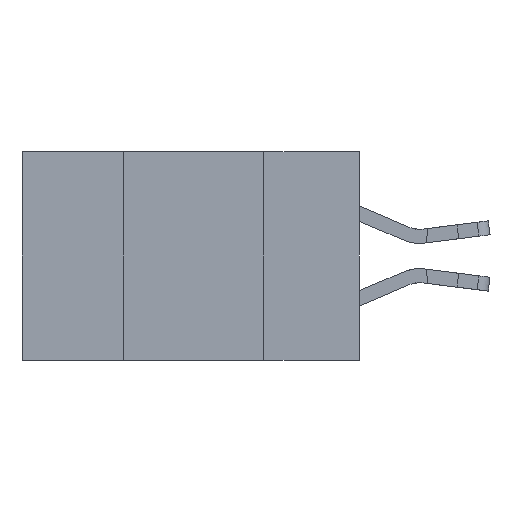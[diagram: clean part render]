
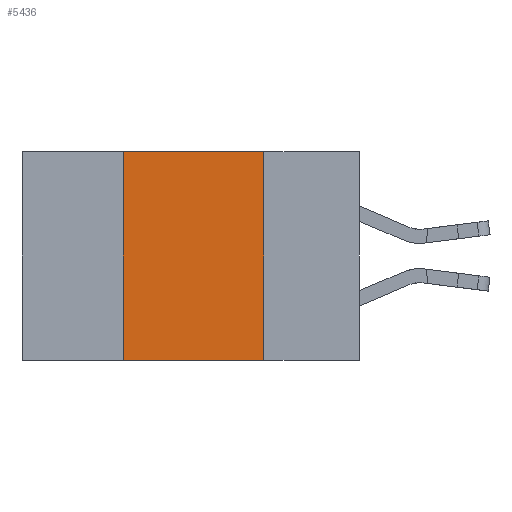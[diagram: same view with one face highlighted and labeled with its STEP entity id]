
A CAD part, left-side view. The second image highlights one B-rep face of the part: STEP entity #5436.
In plain terms, the highlighted planar face has unit normal (-1, 0, 0).
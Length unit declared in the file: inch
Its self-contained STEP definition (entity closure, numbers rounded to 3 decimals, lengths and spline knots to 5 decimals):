
#478 = CARTESIAN_POINT ( 'NONE',  ( 0., 0.17, -0.37 ) ) ;
#2420 = AXIS2_PLACEMENT_3D ( 'NONE', #10141, #10089, #15312 ) ;
#3074 = LINE ( 'NONE', #9071, #9560 ) ;
#3492 = CARTESIAN_POINT ( 'NONE',  ( 0., 0.42, -0.37 ) ) ;
#3863 = VECTOR ( 'NONE', #12169, 39.37008 ) ;
#4345 = EDGE_CURVE ( 'NONE', #14969, #10926, #3074, .T. ) ;
#5436 = ADVANCED_FACE ( 'NONE', ( #9960 ), #6864, .F. ) ;
#5813 = DIRECTION ( 'NONE',  ( 0., 0., -1. ) ) ;
#5998 = DIRECTION ( 'NONE',  ( 0., 0., 1. ) ) ;
#6363 = EDGE_CURVE ( 'NONE', #10428, #10926, #6857, .T. ) ;
#6839 = LINE ( 'NONE', #10558, #16037 ) ;
#6857 = LINE ( 'NONE', #7007, #3863 ) ;
#6864 = PLANE ( 'NONE',  #2420 ) ;
#6871 = EDGE_CURVE ( 'NONE', #11516, #14969, #6839, .T. ) ;
#7007 = CARTESIAN_POINT ( 'NONE',  ( 0., 0.6, -0.37 ) ) ;
#7735 = VECTOR ( 'NONE', #5998, 39.37008 ) ;
#8259 = CARTESIAN_POINT ( 'NONE',  ( 0., 0.17, 0. ) ) ;
#8646 = EDGE_LOOP ( 'NONE', ( #16294, #10387, #9596, #15036 ) ) ;
#9071 = CARTESIAN_POINT ( 'NONE',  ( 0., 0.17, 0. ) ) ;
#9256 = DIRECTION ( 'NONE',  ( 0., -1., 0. ) ) ;
#9560 = VECTOR ( 'NONE', #5813, 39.37008 ) ;
#9596 = ORIENTED_EDGE ( 'NONE', *, *, #9748, .F. ) ;
#9748 = EDGE_CURVE ( 'NONE', #10428, #11516, #11154, .T. ) ;
#9960 = FACE_OUTER_BOUND ( 'NONE', #8646, .T. ) ;
#10089 = DIRECTION ( 'NONE',  ( 1., 0., 0. ) ) ;
#10141 = CARTESIAN_POINT ( 'NONE',  ( 0., 0.6, 0. ) ) ;
#10387 = ORIENTED_EDGE ( 'NONE', *, *, #6871, .F. ) ;
#10428 = VERTEX_POINT ( 'NONE', #3492 ) ;
#10558 = CARTESIAN_POINT ( 'NONE',  ( 0., 0.6, 0. ) ) ;
#10926 = VERTEX_POINT ( 'NONE', #478 ) ;
#11154 = LINE ( 'NONE', #14858, #7735 ) ;
#11516 = VERTEX_POINT ( 'NONE', #15740 ) ;
#12169 = DIRECTION ( 'NONE',  ( 0., -1., 0. ) ) ;
#14858 = CARTESIAN_POINT ( 'NONE',  ( 0., 0.42, 0. ) ) ;
#14969 = VERTEX_POINT ( 'NONE', #8259 ) ;
#15036 = ORIENTED_EDGE ( 'NONE', *, *, #6363, .T. ) ;
#15312 = DIRECTION ( 'NONE',  ( 0., 0., -1. ) ) ;
#15740 = CARTESIAN_POINT ( 'NONE',  ( 0., 0.42, 0. ) ) ;
#16037 = VECTOR ( 'NONE', #9256, 39.37008 ) ;
#16294 = ORIENTED_EDGE ( 'NONE', *, *, #4345, .F. ) ;
